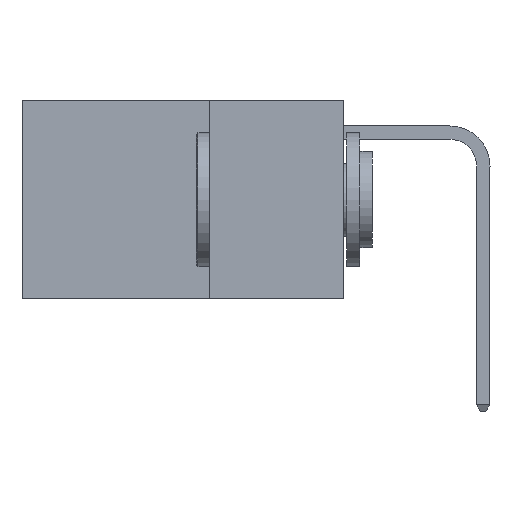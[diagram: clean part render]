
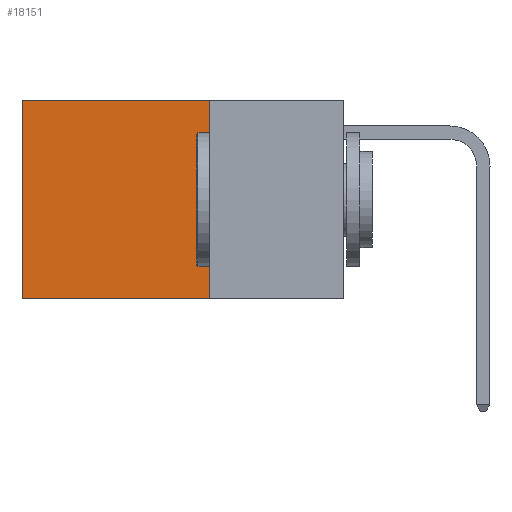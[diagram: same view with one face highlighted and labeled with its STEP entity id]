
A CAD part, left-side view. The second image highlights one B-rep face of the part: STEP entity #18151.
In plain terms, the highlighted planar face has unit normal (-1, 0, 0).
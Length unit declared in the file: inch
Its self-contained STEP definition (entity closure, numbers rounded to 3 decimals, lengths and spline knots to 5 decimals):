
#249 = LINE ( 'NONE', #14183, #4301 ) ;
#1840 = EDGE_CURVE ( 'NONE', #17555, #15260, #6915, .T. ) ;
#2262 = ORIENTED_EDGE ( 'NONE', *, *, #6124, .F. ) ;
#2294 = VECTOR ( 'NONE', #12923, 39.37008 ) ;
#2473 = EDGE_CURVE ( 'NONE', #15260, #10570, #17233, .T. ) ;
#4163 = VECTOR ( 'NONE', #14664, 39.37008 ) ;
#4301 = VECTOR ( 'NONE', #20769, 39.37008 ) ;
#6059 = ORIENTED_EDGE ( 'NONE', *, *, #2473, .T. ) ;
#6124 = EDGE_CURVE ( 'NONE', #17555, #18703, #249, .T. ) ;
#6915 = LINE ( 'NONE', #13492, #2294 ) ;
#7241 = EDGE_CURVE ( 'NONE', #18703, #10570, #7971, .T. ) ;
#7680 = CARTESIAN_POINT ( 'NONE',  ( 0.2625, 0.25, -0.37 ) ) ;
#7729 = CARTESIAN_POINT ( 'NONE',  ( 0.2625, 0.6, 0. ) ) ;
#7928 = DIRECTION ( 'NONE',  ( 1., 0., 0. ) ) ;
#7971 = LINE ( 'NONE', #8606, #12539 ) ;
#8606 = CARTESIAN_POINT ( 'NONE',  ( 0.2625, 0.25, -0.37 ) ) ;
#9675 = ORIENTED_EDGE ( 'NONE', *, *, #7241, .F. ) ;
#10414 = CARTESIAN_POINT ( 'NONE',  ( 0.2625, 0.25, 0. ) ) ;
#10570 = VERTEX_POINT ( 'NONE', #12870 ) ;
#11616 = EDGE_LOOP ( 'NONE', ( #6059, #9675, #2262, #13143 ) ) ;
#12539 = VECTOR ( 'NONE', #20391, 39.37008 ) ;
#12870 = CARTESIAN_POINT ( 'NONE',  ( 0.2625, 0.6, -0.37 ) ) ;
#12923 = DIRECTION ( 'NONE',  ( 0., 1., 0. ) ) ;
#13143 = ORIENTED_EDGE ( 'NONE', *, *, #1840, .T. ) ;
#13492 = CARTESIAN_POINT ( 'NONE',  ( 0.2625, 0.25, 0. ) ) ;
#14183 = CARTESIAN_POINT ( 'NONE',  ( 0.2625, 0.25, 0. ) ) ;
#14664 = DIRECTION ( 'NONE',  ( 0., 0., -1. ) ) ;
#14707 = PLANE ( 'NONE',  #15058 ) ;
#14728 = CARTESIAN_POINT ( 'NONE',  ( 0.2625, 0.6, 0. ) ) ;
#15058 = AXIS2_PLACEMENT_3D ( 'NONE', #18073, #7928, #19738 ) ;
#15260 = VERTEX_POINT ( 'NONE', #7729 ) ;
#15352 = FACE_OUTER_BOUND ( 'NONE', #11616, .T. ) ;
#17233 = LINE ( 'NONE', #14728, #4163 ) ;
#17555 = VERTEX_POINT ( 'NONE', #10414 ) ;
#18073 = CARTESIAN_POINT ( 'NONE',  ( 0.2625, 0.25, 0. ) ) ;
#18151 = ADVANCED_FACE ( 'NONE', ( #15352 ), #14707, .F. ) ;
#18703 = VERTEX_POINT ( 'NONE', #7680 ) ;
#19738 = DIRECTION ( 'NONE',  ( 0., 0., -1. ) ) ;
#20391 = DIRECTION ( 'NONE',  ( 0., 1., 0. ) ) ;
#20769 = DIRECTION ( 'NONE',  ( 0., 0., -1. ) ) ;
